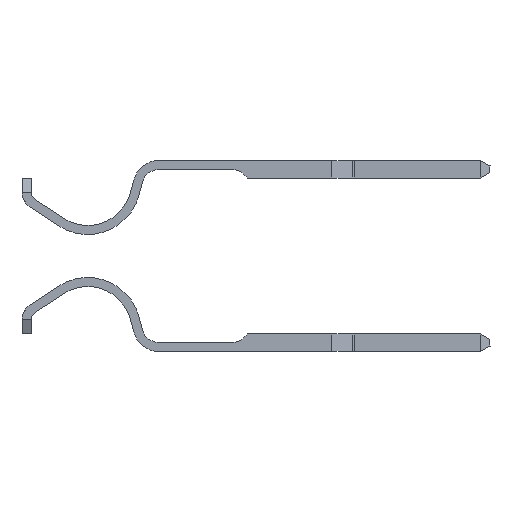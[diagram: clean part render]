
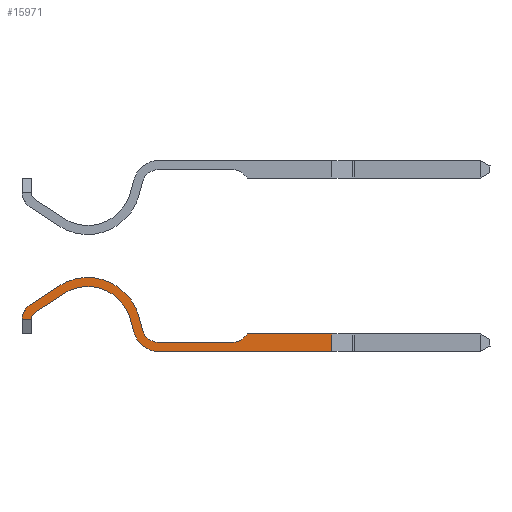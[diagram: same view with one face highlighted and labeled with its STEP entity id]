
A CAD part, left-side view. The second image highlights one B-rep face of the part: STEP entity #15971.
In plain terms, the highlighted face is planar.
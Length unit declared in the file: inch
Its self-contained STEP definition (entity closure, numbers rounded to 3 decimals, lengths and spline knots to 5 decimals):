
#457 = DIRECTION ( 'NONE',  ( -1., 0., 0. ) ) ;
#725 = CARTESIAN_POINT ( 'NONE',  ( 0.33, 0.0255, 0.025 ) ) ;
#807 = ORIENTED_EDGE ( 'NONE', *, *, #21819, .F. ) ;
#1011 = DIRECTION ( 'NONE',  ( 0.836, 0.549, 0. ) ) ;
#1163 = CARTESIAN_POINT ( 'NONE',  ( 0.14518, 0.07966, 0.025 ) ) ;
#1361 = ORIENTED_EDGE ( 'NONE', *, *, #9485, .F. ) ;
#1600 = EDGE_CURVE ( 'NONE', #12105, #16432, #23221, .T. ) ;
#2029 = DIRECTION ( 'NONE',  ( 0., 0., -1. ) ) ;
#2105 = DIRECTION ( 'NONE',  ( -1., 0., 0. ) ) ;
#2186 = EDGE_CURVE ( 'NONE', #13623, #12105, #16306, .T. ) ;
#2290 = CARTESIAN_POINT ( 'NONE',  ( 0.15231, 0.06879, 0.025 ) ) ;
#2373 = ORIENTED_EDGE ( 'NONE', *, *, #18931, .F. ) ;
#2386 = CARTESIAN_POINT ( 'NONE',  ( 0.13322, 0.058, 0.025 ) ) ;
#2866 = CARTESIAN_POINT ( 'NONE',  ( 0.28917, 0.05955, 0.025 ) ) ;
#3075 = CARTESIAN_POINT ( 'NONE',  ( 0.30169, 0.06304, 0.025 ) ) ;
#3098 = EDGE_CURVE ( 'NONE', #4302, #5326, #19040, .T. ) ;
#3120 = CARTESIAN_POINT ( 'NONE',  ( 0.43721, 0.04723, 0.025 ) ) ;
#3153 = CARTESIAN_POINT ( 'NONE',  ( 0.30736, 0.04269, 0.025 ) ) ;
#3719 = VERTEX_POINT ( 'NONE', #725 ) ;
#3898 = ORIENTED_EDGE ( 'NONE', *, *, #10317, .T. ) ;
#4302 = VERTEX_POINT ( 'NONE', #12150 ) ;
#4305 = VERTEX_POINT ( 'NONE', #19516 ) ;
#4441 = DIRECTION ( 'NONE',  ( 0., 0., -1. ) ) ;
#4638 = CARTESIAN_POINT ( 'NONE',  ( 0.45821, 0.0375, 0.025 ) ) ;
#4824 = VECTOR ( 'NONE', #15739, 39.37008 ) ;
#4830 = AXIS2_PLACEMENT_3D ( 'NONE', #13739, #21466, #21096 ) ;
#4833 = AXIS2_PLACEMENT_3D ( 'NONE', #12832, #7164, #21896 ) ;
#5135 = LINE ( 'NONE', #14289, #19170 ) ;
#5326 = VERTEX_POINT ( 'NONE', #2290 ) ;
#5455 = CARTESIAN_POINT ( 'NONE',  ( 0.29484, 0.0392, 0.025 ) ) ;
#5701 = CARTESIAN_POINT ( 'NONE',  ( 0.58021, 0.0375, 0.025 ) ) ;
#5982 = CARTESIAN_POINT ( 'NONE',  ( 0.45258, 0.03186, 0.025 ) ) ;
#6053 = ORIENTED_EDGE ( 'NONE', *, *, #7683, .T. ) ;
#6168 = VECTOR ( 'NONE', #10484, 39.37008 ) ;
#6314 = LINE ( 'NONE', #18861, #18877 ) ;
#6757 = EDGE_CURVE ( 'NONE', #16274, #13375, #22958, .T. ) ;
#6860 = CARTESIAN_POINT ( 'NONE',  ( 0.30169, 0.06304, 0.025 ) ) ;
#6872 = ORIENTED_EDGE ( 'NONE', *, *, #2186, .T. ) ;
#7035 = ORIENTED_EDGE ( 'NONE', *, *, #7441, .T. ) ;
#7164 = DIRECTION ( 'NONE',  ( 0., 0., 1. ) ) ;
#7200 = DIRECTION ( 'NONE',  ( 0., 0., -1. ) ) ;
#7441 = EDGE_CURVE ( 'NONE', #4305, #7600, #5135, .T. ) ;
#7600 = VERTEX_POINT ( 'NONE', #14775 ) ;
#7683 = EDGE_CURVE ( 'NONE', #20197, #4305, #11082, .T. ) ;
#7847 = ORIENTED_EDGE ( 'NONE', *, *, #19607, .F. ) ;
#7853 = AXIS2_PLACEMENT_3D ( 'NONE', #14987, #16693, #2105 ) ;
#8030 = EDGE_CURVE ( 'NONE', #9710, #20162, #13802, .T. ) ;
#8523 = ORIENTED_EDGE ( 'NONE', *, *, #1600, .T. ) ;
#9412 = ORIENTED_EDGE ( 'NONE', *, *, #14481, .T. ) ;
#9485 = EDGE_CURVE ( 'NONE', #20162, #17107, #10719, .T. ) ;
#9543 = DIRECTION ( 'NONE',  ( 0., 0., -1. ) ) ;
#9584 = VECTOR ( 'NONE', #18652, 39.37008 ) ;
#9710 = VERTEX_POINT ( 'NONE', #18410 ) ;
#9715 = CARTESIAN_POINT ( 'NONE',  ( 0.28917, 0.05955, 0.025 ) ) ;
#10045 = DIRECTION ( 'NONE',  ( 1., 0., 0. ) ) ;
#10274 = VERTEX_POINT ( 'NONE', #15612 ) ;
#10317 = EDGE_CURVE ( 'NONE', #14689, #4302, #6314, .T. ) ;
#10484 = DIRECTION ( 'NONE',  ( 0.836, 0.549, 0. ) ) ;
#10509 = EDGE_CURVE ( 'NONE', #5326, #16274, #23445, .T. ) ;
#10719 = LINE ( 'NONE', #6860, #12275 ) ;
#10939 = AXIS2_PLACEMENT_3D ( 'NONE', #17344, #4441, #22914 ) ;
#11010 = LINE ( 'NONE', #5701, #11648 ) ;
#11069 = CARTESIAN_POINT ( 'NONE',  ( 0.095, 0.025, 0.025 ) ) ;
#11082 = CIRCLE ( 'NONE', #21107, 0.0365 ) ;
#11292 = LINE ( 'NONE', #9715, #9584 ) ;
#11331 = VERTEX_POINT ( 'NONE', #1163 ) ;
#11614 = DIRECTION ( 'NONE',  ( 0., 0., 1. ) ) ;
#11648 = VECTOR ( 'NONE', #23815, 39.37008 ) ;
#11720 = CARTESIAN_POINT ( 'NONE',  ( 0.58021, 0.0375, 0.025 ) ) ;
#12105 = VERTEX_POINT ( 'NONE', #17274 ) ;
#12150 = CARTESIAN_POINT ( 'NONE',  ( 0.14622, 0.058, 0.025 ) ) ;
#12181 = LINE ( 'NONE', #21603, #6168 ) ;
#12242 = DIRECTION ( 'NONE',  ( 1., 0., 0. ) ) ;
#12275 = VECTOR ( 'NONE', #21727, 39.37008 ) ;
#12832 = CARTESIAN_POINT ( 'NONE',  ( 0.33, 0.049, 0.025 ) ) ;
#13003 = DIRECTION ( 'NONE',  ( 1., 0., 0. ) ) ;
#13375 = VERTEX_POINT ( 'NONE', #2866 ) ;
#13623 = VERTEX_POINT ( 'NONE', #11720 ) ;
#13739 = CARTESIAN_POINT ( 'NONE',  ( 0.228, 0.0425, 0.025 ) ) ;
#13802 = CIRCLE ( 'NONE', #18407, 0.0765 ) ;
#13950 = CIRCLE ( 'NONE', #15491, 0.02173 ) ;
#14100 = ORIENTED_EDGE ( 'NONE', *, *, #15497, .F. ) ;
#14289 = CARTESIAN_POINT ( 'NONE',  ( 0.33, 0.0125, 0.025 ) ) ;
#14481 = EDGE_CURVE ( 'NONE', #16432, #10274, #13950, .T. ) ;
#14689 = VERTEX_POINT ( 'NONE', #2386 ) ;
#14775 = CARTESIAN_POINT ( 'NONE',  ( 0.58021, 0.0125, 0.025 ) ) ;
#14821 = LINE ( 'NONE', #18427, #17116 ) ;
#14863 = DIRECTION ( 'NONE',  ( -1., 0., 0. ) ) ;
#14987 = CARTESIAN_POINT ( 'NONE',  ( 0.15971, 0.0575, 0.025 ) ) ;
#15045 = FACE_OUTER_BOUND ( 'NONE', #20770, .T. ) ;
#15287 = PLANE ( 'NONE',  #21719 ) ;
#15368 = DIRECTION ( 'NONE',  ( 1., 0., 0. ) ) ;
#15491 = AXIS2_PLACEMENT_3D ( 'NONE', #3120, #7200, #16263 ) ;
#15497 = EDGE_CURVE ( 'NONE', #13623, #7600, #11010, .T. ) ;
#15559 = ORIENTED_EDGE ( 'NONE', *, *, #6757, .T. ) ;
#15612 = CARTESIAN_POINT ( 'NONE',  ( 0.43721, 0.0255, 0.025 ) ) ;
#15739 = DIRECTION ( 'NONE',  ( -0.707, -0.707, 0. ) ) ;
#15971 = ADVANCED_FACE ( 'NONE', ( #15045 ), #15287, .F. ) ;
#16263 = DIRECTION ( 'NONE',  ( 1., 0., 0. ) ) ;
#16274 = VERTEX_POINT ( 'NONE', #21912 ) ;
#16306 = LINE ( 'NONE', #23676, #17155 ) ;
#16313 = ORIENTED_EDGE ( 'NONE', *, *, #3098, .T. ) ;
#16387 = CIRCLE ( 'NONE', #4833, 0.0235 ) ;
#16432 = VERTEX_POINT ( 'NONE', #5982 ) ;
#16693 = DIRECTION ( 'NONE',  ( 0., 0., -1. ) ) ;
#17107 = VERTEX_POINT ( 'NONE', #3153 ) ;
#17116 = VECTOR ( 'NONE', #13003, 39.37008 ) ;
#17155 = VECTOR ( 'NONE', #18453, 39.37008 ) ;
#17274 = CARTESIAN_POINT ( 'NONE',  ( 0.45821, 0.0375, 0.025 ) ) ;
#17344 = CARTESIAN_POINT ( 'NONE',  ( 0.15971, 0.0575, 0.025 ) ) ;
#17770 = CARTESIAN_POINT ( 'NONE',  ( 0.15231, 0.06879, 0.025 ) ) ;
#18407 = AXIS2_PLACEMENT_3D ( 'NONE', #18592, #9543, #14863 ) ;
#18410 = CARTESIAN_POINT ( 'NONE',  ( 0.18604, 0.10646, 0.025 ) ) ;
#18427 = CARTESIAN_POINT ( 'NONE',  ( 0.33, 0.0255, 0.025 ) ) ;
#18453 = DIRECTION ( 'NONE',  ( -1., 0., 0. ) ) ;
#18592 = CARTESIAN_POINT ( 'NONE',  ( 0.228, 0.0425, 0.025 ) ) ;
#18650 = CIRCLE ( 'NONE', #10939, 0.0265 ) ;
#18652 = DIRECTION ( 'NONE',  ( 0.268, -0.963, 0. ) ) ;
#18850 = EDGE_CURVE ( 'NONE', #3719, #10274, #14821, .T. ) ;
#18861 = CARTESIAN_POINT ( 'NONE',  ( 0.14621, 0.058, 0.025 ) ) ;
#18877 = VECTOR ( 'NONE', #10045, 39.37008 ) ;
#18931 = EDGE_CURVE ( 'NONE', #14689, #11331, #18650, .T. ) ;
#19040 = CIRCLE ( 'NONE', #7853, 0.0135 ) ;
#19170 = VECTOR ( 'NONE', #12242, 39.37008 ) ;
#19516 = CARTESIAN_POINT ( 'NONE',  ( 0.33, 0.0125, 0.025 ) ) ;
#19607 = EDGE_CURVE ( 'NONE', #17107, #3719, #16387, .T. ) ;
#19731 = ORIENTED_EDGE ( 'NONE', *, *, #18850, .F. ) ;
#20162 = VERTEX_POINT ( 'NONE', #3075 ) ;
#20197 = VERTEX_POINT ( 'NONE', #5455 ) ;
#20770 = EDGE_LOOP ( 'NONE', ( #2373, #3898, #16313, #22434, #15559, #20842, #6053, #7035, #14100, #6872, #8523, #9412, #19731, #7847, #1361, #21228, #807 ) ) ;
#20842 = ORIENTED_EDGE ( 'NONE', *, *, #22557, .T. ) ;
#21096 = DIRECTION ( 'NONE',  ( -1., 0., 0. ) ) ;
#21107 = AXIS2_PLACEMENT_3D ( 'NONE', #22745, #11614, #15368 ) ;
#21228 = ORIENTED_EDGE ( 'NONE', *, *, #8030, .F. ) ;
#21466 = DIRECTION ( 'NONE',  ( 0., 0., -1. ) ) ;
#21603 = CARTESIAN_POINT ( 'NONE',  ( 0.14518, 0.07966, 0.025 ) ) ;
#21719 = AXIS2_PLACEMENT_3D ( 'NONE', #11069, #2029, #457 ) ;
#21727 = DIRECTION ( 'NONE',  ( 0.268, -0.963, 0. ) ) ;
#21819 = EDGE_CURVE ( 'NONE', #11331, #9710, #12181, .T. ) ;
#21896 = DIRECTION ( 'NONE',  ( 1., 0., 0. ) ) ;
#21912 = CARTESIAN_POINT ( 'NONE',  ( 0.19317, 0.09559, 0.025 ) ) ;
#21960 = VECTOR ( 'NONE', #1011, 39.37008 ) ;
#22434 = ORIENTED_EDGE ( 'NONE', *, *, #10509, .T. ) ;
#22557 = EDGE_CURVE ( 'NONE', #13375, #20197, #11292, .T. ) ;
#22745 = CARTESIAN_POINT ( 'NONE',  ( 0.33, 0.049, 0.025 ) ) ;
#22914 = DIRECTION ( 'NONE',  ( -1., 0., 0. ) ) ;
#22958 = CIRCLE ( 'NONE', #4830, 0.0635 ) ;
#23221 = LINE ( 'NONE', #4638, #4824 ) ;
#23445 = LINE ( 'NONE', #17770, #21960 ) ;
#23676 = CARTESIAN_POINT ( 'NONE',  ( 0.45821, 0.0375, 0.025 ) ) ;
#23815 = DIRECTION ( 'NONE',  ( 0., -1., 0. ) ) ;
